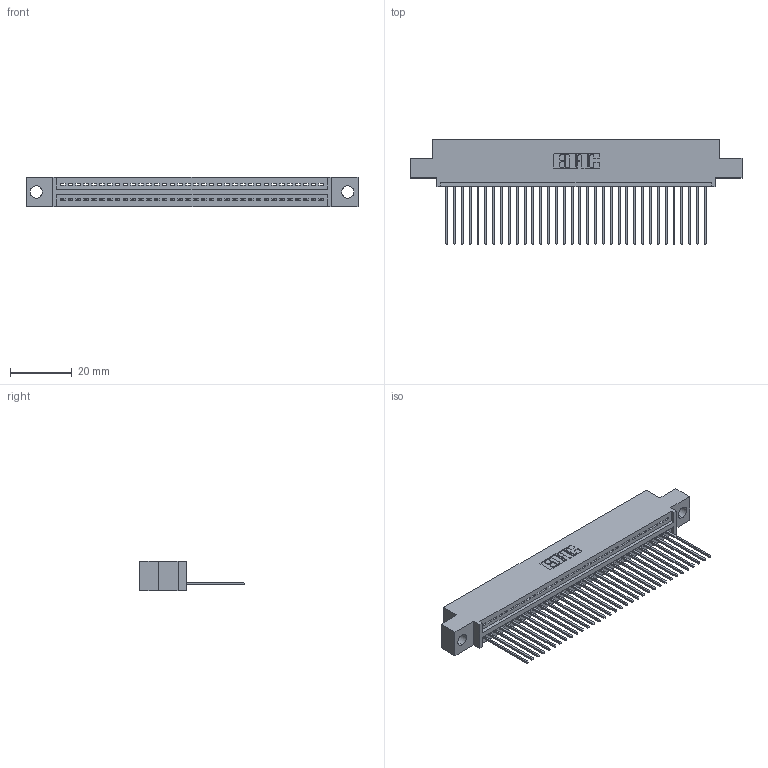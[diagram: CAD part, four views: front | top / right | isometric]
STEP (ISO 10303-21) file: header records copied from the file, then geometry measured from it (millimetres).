
FILE_DESCRIPTION (( 'STEP AP203' ), '1' );
FILE_NAME ('345-034-541-404.STEP', '2021-05-26T14:46:19', ( '' ), ( '' ), 'SwSTEP 2.0', 'SolidWorks 2020', '' );
FILE_SCHEMA (( 'CONFIG_CONTROL_DESIGN' ));
Length unit declared in the file: inch
Products named in the file (3): 345-292-001_345-293-141; 345-034-541-404; 345 Part_0.110 Offset - 0.156 Dia-TI
Assembly tree (35 placements, depth 2):
  345-034-541-404
    345 Part_0.110 Offset - 0.156 Dia-TI
    345-292-001_345-293-141  x34
Bounding box: 107.57 x 33.96 x 9.4 mm (x, y, z)
Volume: 10084.4 mm3; surface area: 13877 mm2
Topology: 35 solids, 35 shells, 2116 faces, 6373 edges, 4202 vertices
Faces by surface type: plane 1458, cylinder 658
Entity records: 27235 total; most frequent: CARTESIAN_POINT 4728, ORIENTED_EDGE 4694, DIRECTION 4139, EDGE_CURVE 2347, LINE 2079, VECTOR 2079, VERTEX_POINT 1562, AXIS2_PLACEMENT_3D 1030
